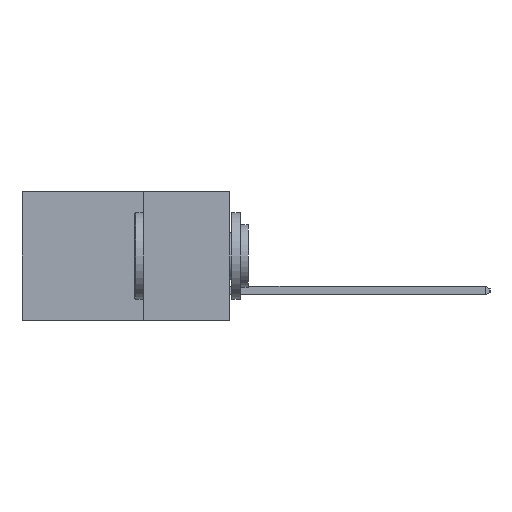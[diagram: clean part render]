
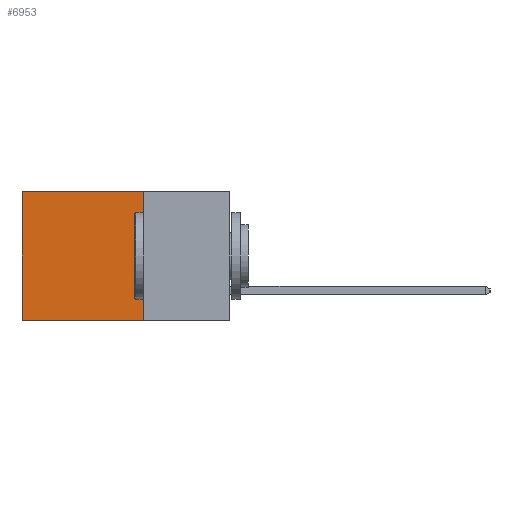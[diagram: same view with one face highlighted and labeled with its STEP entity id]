
A CAD part, left-side view. The second image highlights one B-rep face of the part: STEP entity #6953.
In plain terms, the highlighted planar face has unit normal (-1, 0, 0).
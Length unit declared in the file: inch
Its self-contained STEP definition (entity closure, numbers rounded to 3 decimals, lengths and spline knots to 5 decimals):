
#1354 = EDGE_CURVE ( 'NONE', #9198, #16857, #6978, .T. ) ;
#1673 = VERTEX_POINT ( 'NONE', #11843 ) ;
#2047 = CARTESIAN_POINT ( 'NONE',  ( 0.298, 0.6, -0.37 ) ) ;
#2049 = EDGE_CURVE ( 'NONE', #1673, #17552, #3189, .T. ) ;
#2749 = EDGE_CURVE ( 'NONE', #16857, #17552, #18144, .T. ) ;
#3189 = LINE ( 'NONE', #13011, #10618 ) ;
#3723 = CARTESIAN_POINT ( 'NONE',  ( 0.298, 0.25, -0.37 ) ) ;
#5580 = CARTESIAN_POINT ( 'NONE',  ( 0.298, 0.25, -0.37 ) ) ;
#6609 = EDGE_LOOP ( 'NONE', ( #11665, #8869, #7352, #15985 ) ) ;
#6924 = VECTOR ( 'NONE', #12649, 39.37008 ) ;
#6953 = ADVANCED_FACE ( 'NONE', ( #14116 ), #16945, .F. ) ;
#6978 = LINE ( 'NONE', #18303, #13683 ) ;
#7352 = ORIENTED_EDGE ( 'NONE', *, *, #1354, .F. ) ;
#7955 = DIRECTION ( 'NONE',  ( 0., 1., 0. ) ) ;
#8869 = ORIENTED_EDGE ( 'NONE', *, *, #2749, .F. ) ;
#9198 = VERTEX_POINT ( 'NONE', #12605 ) ;
#10618 = VECTOR ( 'NONE', #13110, 39.37008 ) ;
#11665 = ORIENTED_EDGE ( 'NONE', *, *, #2049, .T. ) ;
#11843 = CARTESIAN_POINT ( 'NONE',  ( 0.298, 0.6, 0. ) ) ;
#12605 = CARTESIAN_POINT ( 'NONE',  ( 0.298, 0.25, 0. ) ) ;
#12649 = DIRECTION ( 'NONE',  ( 0., 1., 0. ) ) ;
#13011 = CARTESIAN_POINT ( 'NONE',  ( 0.298, 0.6, 0. ) ) ;
#13110 = DIRECTION ( 'NONE',  ( 0., 0., -1. ) ) ;
#13683 = VECTOR ( 'NONE', #18713, 39.37008 ) ;
#14116 = FACE_OUTER_BOUND ( 'NONE', #6609, .T. ) ;
#14675 = AXIS2_PLACEMENT_3D ( 'NONE', #16966, #16908, #16863 ) ;
#15448 = LINE ( 'NONE', #16366, #18676 ) ;
#15985 = ORIENTED_EDGE ( 'NONE', *, *, #17233, .T. ) ;
#16366 = CARTESIAN_POINT ( 'NONE',  ( 0.298, 0.25, 0. ) ) ;
#16857 = VERTEX_POINT ( 'NONE', #5580 ) ;
#16863 = DIRECTION ( 'NONE',  ( 0., 0., -1. ) ) ;
#16908 = DIRECTION ( 'NONE',  ( 1., 0., 0. ) ) ;
#16945 = PLANE ( 'NONE',  #14675 ) ;
#16966 = CARTESIAN_POINT ( 'NONE',  ( 0.298, 0.25, 0. ) ) ;
#17233 = EDGE_CURVE ( 'NONE', #9198, #1673, #15448, .T. ) ;
#17552 = VERTEX_POINT ( 'NONE', #2047 ) ;
#18144 = LINE ( 'NONE', #3723, #6924 ) ;
#18303 = CARTESIAN_POINT ( 'NONE',  ( 0.298, 0.25, 0. ) ) ;
#18676 = VECTOR ( 'NONE', #7955, 39.37008 ) ;
#18713 = DIRECTION ( 'NONE',  ( 0., 0., -1. ) ) ;
